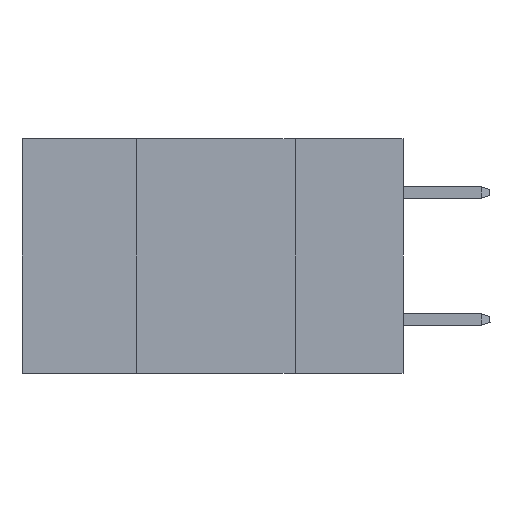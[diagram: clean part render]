
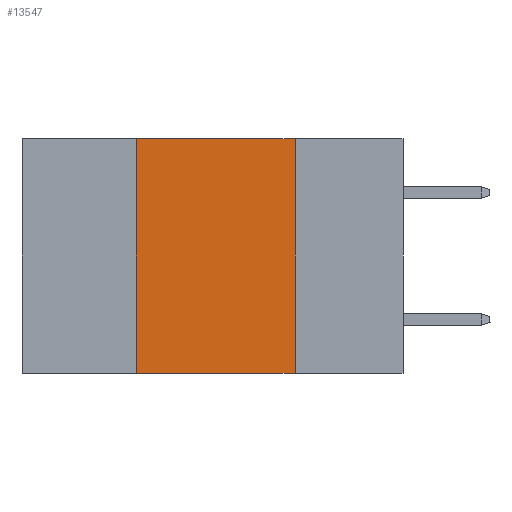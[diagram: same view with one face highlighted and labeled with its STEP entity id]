
A CAD part, left-side view. The second image highlights one B-rep face of the part: STEP entity #13547.
In plain terms, the highlighted planar face has unit normal (-1, 0, 0).
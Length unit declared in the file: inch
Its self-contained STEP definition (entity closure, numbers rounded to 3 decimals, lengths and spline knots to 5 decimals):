
#41 = EDGE_CURVE ( 'NONE', #3670, #5747, #2916, .T. ) ;
#375 = DIRECTION ( 'NONE',  ( 0., 0., -1. ) ) ;
#451 = ORIENTED_EDGE ( 'NONE', *, *, #7592, .F. ) ;
#572 = ORIENTED_EDGE ( 'NONE', *, *, #3436, .F. ) ;
#859 = CARTESIAN_POINT ( 'NONE',  ( 0., 0.42, -0.37 ) ) ;
#1834 = CARTESIAN_POINT ( 'NONE',  ( 0., 0.6, -0.37 ) ) ;
#2049 = DIRECTION ( 'NONE',  ( 0., -1., 0. ) ) ;
#2775 = EDGE_CURVE ( 'NONE', #7583, #10557, #7192, .T. ) ;
#2916 = LINE ( 'NONE', #6388, #13476 ) ;
#3235 = FACE_OUTER_BOUND ( 'NONE', #5667, .T. ) ;
#3436 = EDGE_CURVE ( 'NONE', #5747, #10557, #4678, .T. ) ;
#3670 = VERTEX_POINT ( 'NONE', #10484 ) ;
#4405 = PLANE ( 'NONE',  #5750 ) ;
#4678 = LINE ( 'NONE', #10271, #11491 ) ;
#5327 = ORIENTED_EDGE ( 'NONE', *, *, #2775, .T. ) ;
#5599 = CARTESIAN_POINT ( 'NONE',  ( 0., 0.42, 0. ) ) ;
#5667 = EDGE_LOOP ( 'NONE', ( #572, #12166, #451, #5327 ) ) ;
#5747 = VERTEX_POINT ( 'NONE', #9487 ) ;
#5750 = AXIS2_PLACEMENT_3D ( 'NONE', #7806, #10068, #9858 ) ;
#6388 = CARTESIAN_POINT ( 'NONE',  ( 0., 0.6, 0. ) ) ;
#7192 = LINE ( 'NONE', #1834, #9454 ) ;
#7583 = VERTEX_POINT ( 'NONE', #859 ) ;
#7592 = EDGE_CURVE ( 'NONE', #7583, #3670, #10099, .T. ) ;
#7806 = CARTESIAN_POINT ( 'NONE',  ( 0., 0.6, 0. ) ) ;
#9358 = CARTESIAN_POINT ( 'NONE',  ( 0., 0.17, -0.37 ) ) ;
#9454 = VECTOR ( 'NONE', #10729, 39.37008 ) ;
#9487 = CARTESIAN_POINT ( 'NONE',  ( 0., 0.17, 0. ) ) ;
#9858 = DIRECTION ( 'NONE',  ( 0., 0., -1. ) ) ;
#9896 = DIRECTION ( 'NONE',  ( 0., 0., 1. ) ) ;
#10068 = DIRECTION ( 'NONE',  ( 1., 0., 0. ) ) ;
#10099 = LINE ( 'NONE', #5599, #13951 ) ;
#10271 = CARTESIAN_POINT ( 'NONE',  ( 0., 0.17, 0. ) ) ;
#10484 = CARTESIAN_POINT ( 'NONE',  ( 0., 0.42, 0. ) ) ;
#10557 = VERTEX_POINT ( 'NONE', #9358 ) ;
#10729 = DIRECTION ( 'NONE',  ( 0., -1., 0. ) ) ;
#11491 = VECTOR ( 'NONE', #375, 39.37008 ) ;
#12166 = ORIENTED_EDGE ( 'NONE', *, *, #41, .F. ) ;
#13476 = VECTOR ( 'NONE', #2049, 39.37008 ) ;
#13547 = ADVANCED_FACE ( 'NONE', ( #3235 ), #4405, .F. ) ;
#13951 = VECTOR ( 'NONE', #9896, 39.37008 ) ;
